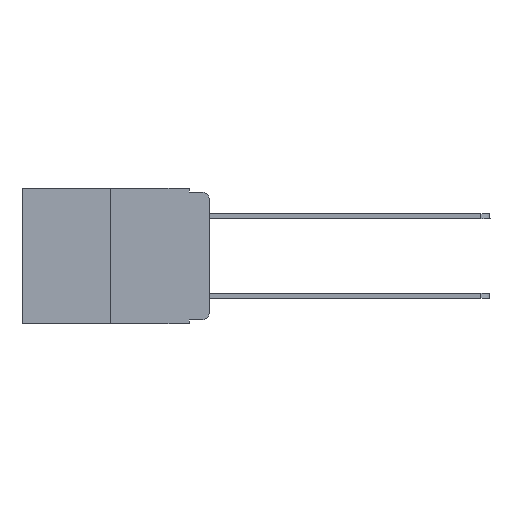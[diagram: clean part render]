
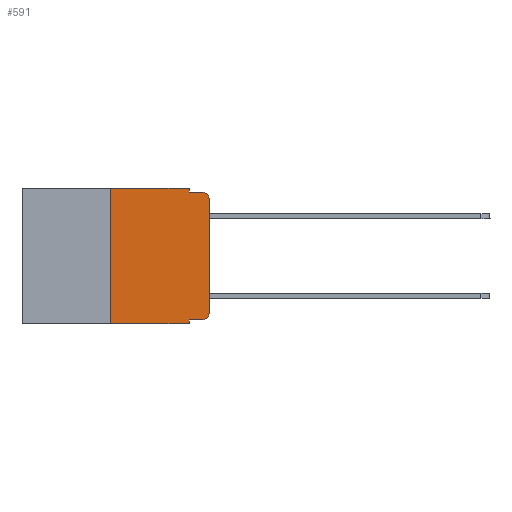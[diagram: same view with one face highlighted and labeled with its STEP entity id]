
A CAD part, left-side view. The second image highlights one B-rep face of the part: STEP entity #591.
In plain terms, the highlighted planar face has unit normal (-1, 0, 0).
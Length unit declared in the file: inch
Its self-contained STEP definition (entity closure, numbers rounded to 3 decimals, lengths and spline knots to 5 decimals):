
#3 = CARTESIAN_POINT ( 'NONE',  ( 0., 0.02, -0.333 ) ) ;
#111 = DIRECTION ( 'NONE',  ( 0., 0., 1. ) ) ;
#193 = CARTESIAN_POINT ( 'NONE',  ( 0., 0.051, -0.01 ) ) ;
#236 = CARTESIAN_POINT ( 'NONE',  ( 0., 0.473, -0.343 ) ) ;
#553 = CARTESIAN_POINT ( 'NONE',  ( 0., 0.051, 0. ) ) ;
#591 = ADVANCED_FACE ( 'NONE', ( #10887 ), #12064, .F. ) ;
#655 = AXIS2_PLACEMENT_3D ( 'NONE', #8630, #5885, #11661 ) ;
#969 = CARTESIAN_POINT ( 'NONE',  ( 0., 0.25, 0. ) ) ;
#1197 = LINE ( 'NONE', #14743, #18022 ) ;
#1366 = EDGE_LOOP ( 'NONE', ( #11986, #7456, #3460, #1431, #18778, #14753, #2912, #10417, #11465, #18689 ) ) ;
#1431 = ORIENTED_EDGE ( 'NONE', *, *, #6687, .F. ) ;
#1501 = VECTOR ( 'NONE', #111, 39.37008 ) ;
#1755 = CIRCLE ( 'NONE', #12095, 0.02 ) ;
#2143 = VERTEX_POINT ( 'NONE', #3 ) ;
#2371 = DIRECTION ( 'NONE',  ( 0., -1., 0. ) ) ;
#2912 = ORIENTED_EDGE ( 'NONE', *, *, #8871, .T. ) ;
#2990 = VECTOR ( 'NONE', #6214, 39.37008 ) ;
#3460 = ORIENTED_EDGE ( 'NONE', *, *, #10304, .F. ) ;
#3621 = EDGE_CURVE ( 'NONE', #9385, #14545, #1197, .T. ) ;
#4183 = DIRECTION ( 'NONE',  ( 0., 0., -1. ) ) ;
#4803 = DIRECTION ( 'NONE',  ( 1., 0., 0. ) ) ;
#5213 = DIRECTION ( 'NONE',  ( 0., -1., 0. ) ) ;
#5409 = CARTESIAN_POINT ( 'NONE',  ( 0., 0.051, -0.333 ) ) ;
#5606 = LINE ( 'NONE', #7073, #5866 ) ;
#5866 = VECTOR ( 'NONE', #2371, 39.37008 ) ;
#5885 = DIRECTION ( 'NONE',  ( -1., 0., 0. ) ) ;
#6214 = DIRECTION ( 'NONE',  ( 0., -1., 0. ) ) ;
#6341 = VERTEX_POINT ( 'NONE', #9693 ) ;
#6416 = VERTEX_POINT ( 'NONE', #15003 ) ;
#6530 = DIRECTION ( 'NONE',  ( 0., 0., -1. ) ) ;
#6687 = EDGE_CURVE ( 'NONE', #14545, #14686, #8010, .T. ) ;
#6880 = LINE ( 'NONE', #5409, #8197 ) ;
#7016 = CARTESIAN_POINT ( 'NONE',  ( 0., 0.25, 0. ) ) ;
#7073 = CARTESIAN_POINT ( 'NONE',  ( 0., 0.051, -0.01 ) ) ;
#7402 = EDGE_CURVE ( 'NONE', #16771, #6416, #16686, .T. ) ;
#7456 = ORIENTED_EDGE ( 'NONE', *, *, #16653, .T. ) ;
#7629 = CARTESIAN_POINT ( 'NONE',  ( 0., 0.051, -0.333 ) ) ;
#7630 = VERTEX_POINT ( 'NONE', #9409 ) ;
#7911 = VECTOR ( 'NONE', #4183, 39.37008 ) ;
#8010 = LINE ( 'NONE', #553, #16201 ) ;
#8197 = VECTOR ( 'NONE', #5213, 39.37008 ) ;
#8630 = CARTESIAN_POINT ( 'NONE',  ( 0., 0.02, -0.03 ) ) ;
#8871 = EDGE_CURVE ( 'NONE', #6341, #7630, #9598, .T. ) ;
#8901 = LINE ( 'NONE', #17816, #7911 ) ;
#9099 = EDGE_CURVE ( 'NONE', #2143, #16771, #1755, .T. ) ;
#9385 = VERTEX_POINT ( 'NONE', #7016 ) ;
#9409 = CARTESIAN_POINT ( 'NONE',  ( 0., 0.051, -0.343 ) ) ;
#9598 = LINE ( 'NONE', #236, #2990 ) ;
#9693 = CARTESIAN_POINT ( 'NONE',  ( 0., 0.25, -0.343 ) ) ;
#10304 = EDGE_CURVE ( 'NONE', #14686, #10881, #5606, .T. ) ;
#10417 = ORIENTED_EDGE ( 'NONE', *, *, #18424, .F. ) ;
#10881 = VERTEX_POINT ( 'NONE', #12586 ) ;
#10887 = FACE_OUTER_BOUND ( 'NONE', #1366, .T. ) ;
#11464 = DIRECTION ( 'NONE',  ( 0., 0., 1. ) ) ;
#11465 = ORIENTED_EDGE ( 'NONE', *, *, #15988, .T. ) ;
#11584 = DIRECTION ( 'NONE',  ( 0., -1., 0. ) ) ;
#11635 = AXIS2_PLACEMENT_3D ( 'NONE', #13563, #4803, #13460 ) ;
#11661 = DIRECTION ( 'NONE',  ( 0., 0., -1. ) ) ;
#11943 = CARTESIAN_POINT ( 'NONE',  ( 0., 0.051, 0. ) ) ;
#11949 = EDGE_CURVE ( 'NONE', #6341, #9385, #14421, .T. ) ;
#11986 = ORIENTED_EDGE ( 'NONE', *, *, #7402, .T. ) ;
#12064 = PLANE ( 'NONE',  #11635 ) ;
#12095 = AXIS2_PLACEMENT_3D ( 'NONE', #16765, #12343, #18309 ) ;
#12194 = VERTEX_POINT ( 'NONE', #7629 ) ;
#12343 = DIRECTION ( 'NONE',  ( -1., 0., 0. ) ) ;
#12586 = CARTESIAN_POINT ( 'NONE',  ( 0., 0.02, -0.01 ) ) ;
#13460 = DIRECTION ( 'NONE',  ( 0., 0., -1. ) ) ;
#13563 = CARTESIAN_POINT ( 'NONE',  ( 0., 0.473, 0. ) ) ;
#14421 = LINE ( 'NONE', #969, #16754 ) ;
#14545 = VERTEX_POINT ( 'NONE', #11943 ) ;
#14686 = VERTEX_POINT ( 'NONE', #193 ) ;
#14743 = CARTESIAN_POINT ( 'NONE',  ( 0., 0.473, 0. ) ) ;
#14753 = ORIENTED_EDGE ( 'NONE', *, *, #11949, .F. ) ;
#15003 = CARTESIAN_POINT ( 'NONE',  ( 0., 0., -0.03 ) ) ;
#15095 = CIRCLE ( 'NONE', #655, 0.02 ) ;
#15223 = CARTESIAN_POINT ( 'NONE',  ( 0., 0., -0.313 ) ) ;
#15234 = CARTESIAN_POINT ( 'NONE',  ( 0., 0., 0. ) ) ;
#15988 = EDGE_CURVE ( 'NONE', #12194, #2143, #6880, .T. ) ;
#16201 = VECTOR ( 'NONE', #6530, 39.37008 ) ;
#16653 = EDGE_CURVE ( 'NONE', #6416, #10881, #15095, .T. ) ;
#16686 = LINE ( 'NONE', #15234, #1501 ) ;
#16754 = VECTOR ( 'NONE', #11464, 39.37008 ) ;
#16765 = CARTESIAN_POINT ( 'NONE',  ( 0., 0.02, -0.313 ) ) ;
#16771 = VERTEX_POINT ( 'NONE', #15223 ) ;
#17816 = CARTESIAN_POINT ( 'NONE',  ( 0., 0.051, 0. ) ) ;
#18022 = VECTOR ( 'NONE', #11584, 39.37008 ) ;
#18309 = DIRECTION ( 'NONE',  ( 0., 0., -1. ) ) ;
#18424 = EDGE_CURVE ( 'NONE', #12194, #7630, #8901, .T. ) ;
#18689 = ORIENTED_EDGE ( 'NONE', *, *, #9099, .T. ) ;
#18778 = ORIENTED_EDGE ( 'NONE', *, *, #3621, .F. ) ;
